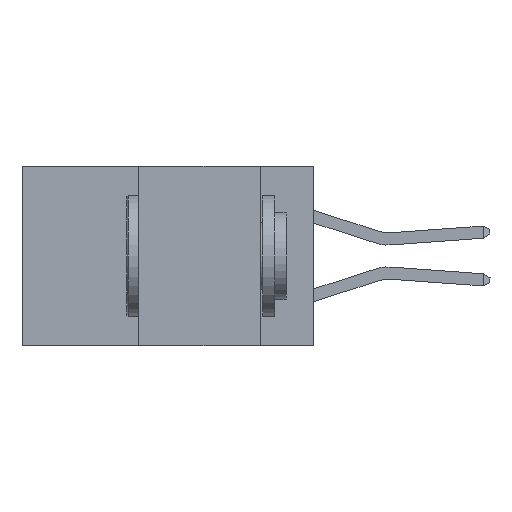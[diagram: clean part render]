
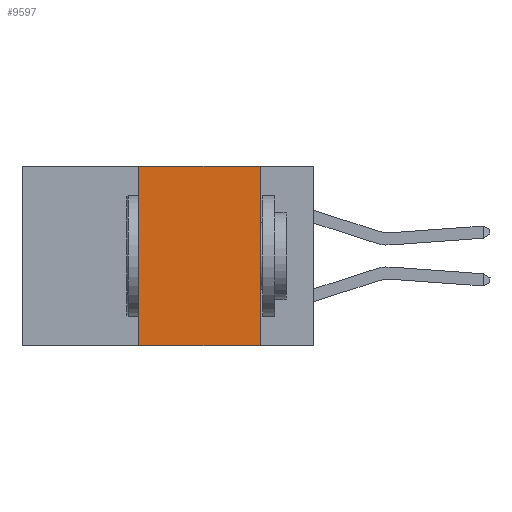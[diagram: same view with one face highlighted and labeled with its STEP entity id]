
A CAD part, left-side view. The second image highlights one B-rep face of the part: STEP entity #9597.
In plain terms, the highlighted planar face has unit normal (-1, 0, 0).
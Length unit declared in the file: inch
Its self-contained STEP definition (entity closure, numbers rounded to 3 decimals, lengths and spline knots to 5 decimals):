
#1172 = CARTESIAN_POINT ( 'NONE',  ( 0., 0.11, 0. ) ) ;
#2138 = DIRECTION ( 'NONE',  ( 0., 0., -1. ) ) ;
#2564 = CARTESIAN_POINT ( 'NONE',  ( 0., 0.36, 0. ) ) ;
#3500 = FACE_OUTER_BOUND ( 'NONE', #25837, .T. ) ;
#5185 = VECTOR ( 'NONE', #11699, 39.37008 ) ;
#5243 = DIRECTION ( 'NONE',  ( 1., 0., 0. ) ) ;
#6200 = ORIENTED_EDGE ( 'NONE', *, *, #35559, .T. ) ;
#6743 = ORIENTED_EDGE ( 'NONE', *, *, #19586, .F. ) ;
#8056 = VERTEX_POINT ( 'NONE', #34824 ) ;
#9597 = ADVANCED_FACE ( 'NONE', ( #3500 ), #32461, .F. ) ;
#9735 = VECTOR ( 'NONE', #10716, 39.37008 ) ;
#10716 = DIRECTION ( 'NONE',  ( 0., 0., 1. ) ) ;
#11474 = CARTESIAN_POINT ( 'NONE',  ( 0., 0.36, -0.37 ) ) ;
#11699 = DIRECTION ( 'NONE',  ( 0., -1., 0. ) ) ;
#13858 = VECTOR ( 'NONE', #33049, 39.37008 ) ;
#14337 = CARTESIAN_POINT ( 'NONE',  ( 0., 0.11, 0. ) ) ;
#14533 = ORIENTED_EDGE ( 'NONE', *, *, #17261, .F. ) ;
#15280 = CARTESIAN_POINT ( 'NONE',  ( 0., 0.36, 0. ) ) ;
#15893 = CARTESIAN_POINT ( 'NONE',  ( 0., 0.6, 0. ) ) ;
#17128 = LINE ( 'NONE', #2564, #9735 ) ;
#17261 = EDGE_CURVE ( 'NONE', #24183, #8056, #23032, .T. ) ;
#18115 = CARTESIAN_POINT ( 'NONE',  ( 0., 0.6, -0.37 ) ) ;
#19586 = EDGE_CURVE ( 'NONE', #25473, #24183, #24218, .T. ) ;
#19644 = VERTEX_POINT ( 'NONE', #11474 ) ;
#22460 = LINE ( 'NONE', #18115, #13858 ) ;
#23032 = LINE ( 'NONE', #14337, #29563 ) ;
#24183 = VERTEX_POINT ( 'NONE', #1172 ) ;
#24218 = LINE ( 'NONE', #30629, #5185 ) ;
#25203 = EDGE_CURVE ( 'NONE', #19644, #25473, #17128, .T. ) ;
#25473 = VERTEX_POINT ( 'NONE', #15280 ) ;
#25837 = EDGE_LOOP ( 'NONE', ( #14533, #6743, #29696, #6200 ) ) ;
#28646 = AXIS2_PLACEMENT_3D ( 'NONE', #15893, #5243, #2138 ) ;
#29563 = VECTOR ( 'NONE', #33713, 39.37008 ) ;
#29696 = ORIENTED_EDGE ( 'NONE', *, *, #25203, .F. ) ;
#30629 = CARTESIAN_POINT ( 'NONE',  ( 0., 0.6, 0. ) ) ;
#32461 = PLANE ( 'NONE',  #28646 ) ;
#33049 = DIRECTION ( 'NONE',  ( 0., -1., 0. ) ) ;
#33713 = DIRECTION ( 'NONE',  ( 0., 0., -1. ) ) ;
#34824 = CARTESIAN_POINT ( 'NONE',  ( 0., 0.11, -0.37 ) ) ;
#35559 = EDGE_CURVE ( 'NONE', #19644, #8056, #22460, .T. ) ;
